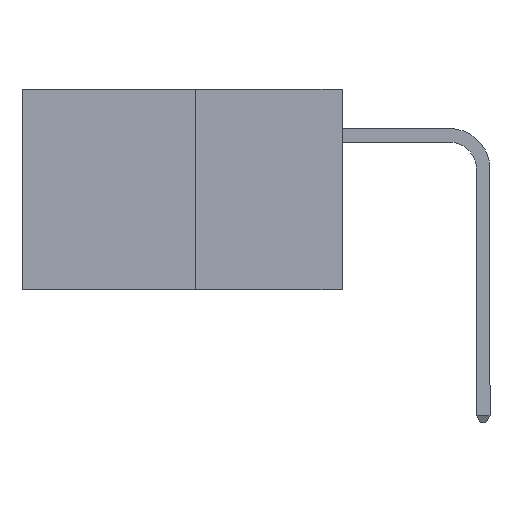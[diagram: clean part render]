
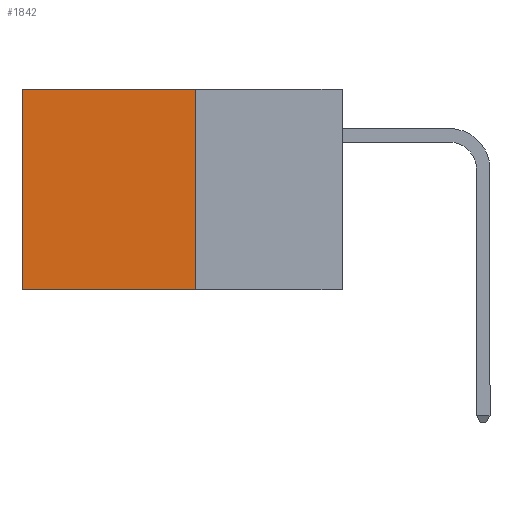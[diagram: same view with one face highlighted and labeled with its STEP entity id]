
A CAD part, left-side view. The second image highlights one B-rep face of the part: STEP entity #1842.
In plain terms, the highlighted planar face has unit normal (-1, 0, 0).
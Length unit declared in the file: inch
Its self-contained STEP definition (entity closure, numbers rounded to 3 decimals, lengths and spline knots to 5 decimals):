
#84 = EDGE_CURVE ( 'NONE', #8713, #3775, #1923, .T. ) ;
#627 = DIRECTION ( 'NONE',  ( 0., 0., -1. ) ) ;
#635 = DIRECTION ( 'NONE',  ( 1., 0., 0. ) ) ;
#693 = PLANE ( 'NONE',  #4722 ) ;
#752 = CARTESIAN_POINT ( 'NONE',  ( 0.277, 0.27, -0.37 ) ) ;
#1280 = ORIENTED_EDGE ( 'NONE', *, *, #2383, .T. ) ;
#1842 = ADVANCED_FACE ( 'NONE', ( #4798 ), #693, .F. ) ;
#1923 = LINE ( 'NONE', #8838, #6191 ) ;
#2383 = EDGE_CURVE ( 'NONE', #7583, #3595, #4410, .T. ) ;
#2433 = DIRECTION ( 'NONE',  ( 0., 1., 0. ) ) ;
#2625 = DIRECTION ( 'NONE',  ( 0., 0., -1. ) ) ;
#2713 = ORIENTED_EDGE ( 'NONE', *, *, #9541, .F. ) ;
#2725 = LINE ( 'NONE', #6598, #4618 ) ;
#3334 = CARTESIAN_POINT ( 'NONE',  ( 0.277, 0.27, 0. ) ) ;
#3595 = VERTEX_POINT ( 'NONE', #7338 ) ;
#3775 = VERTEX_POINT ( 'NONE', #6425 ) ;
#3900 = VECTOR ( 'NONE', #8499, 39.37008 ) ;
#4402 = EDGE_LOOP ( 'NONE', ( #5760, #10307, #2713, #1280 ) ) ;
#4410 = LINE ( 'NONE', #8507, #8310 ) ;
#4618 = VECTOR ( 'NONE', #2625, 39.37008 ) ;
#4722 = AXIS2_PLACEMENT_3D ( 'NONE', #752, #635, #627 ) ;
#4798 = FACE_OUTER_BOUND ( 'NONE', #4402, .T. ) ;
#5760 = ORIENTED_EDGE ( 'NONE', *, *, #7963, .T. ) ;
#6191 = VECTOR ( 'NONE', #2433, 39.37008 ) ;
#6425 = CARTESIAN_POINT ( 'NONE',  ( 0.277, 0.59, -0.37 ) ) ;
#6598 = CARTESIAN_POINT ( 'NONE',  ( 0.277, 0.27, -0.37 ) ) ;
#7089 = CARTESIAN_POINT ( 'NONE',  ( 0.277, 0.27, -0.37 ) ) ;
#7338 = CARTESIAN_POINT ( 'NONE',  ( 0.277, 0.59, 0. ) ) ;
#7583 = VERTEX_POINT ( 'NONE', #3334 ) ;
#7963 = EDGE_CURVE ( 'NONE', #3595, #3775, #8068, .T. ) ;
#8068 = LINE ( 'NONE', #9279, #3900 ) ;
#8310 = VECTOR ( 'NONE', #8554, 39.37008 ) ;
#8499 = DIRECTION ( 'NONE',  ( 0., 0., -1. ) ) ;
#8507 = CARTESIAN_POINT ( 'NONE',  ( 0.277, 0.27, 0. ) ) ;
#8554 = DIRECTION ( 'NONE',  ( 0., 1., 0. ) ) ;
#8713 = VERTEX_POINT ( 'NONE', #7089 ) ;
#8838 = CARTESIAN_POINT ( 'NONE',  ( 0.277, 0.27, -0.37 ) ) ;
#9279 = CARTESIAN_POINT ( 'NONE',  ( 0.277, 0.59, -0.37 ) ) ;
#9541 = EDGE_CURVE ( 'NONE', #7583, #8713, #2725, .T. ) ;
#10307 = ORIENTED_EDGE ( 'NONE', *, *, #84, .F. ) ;
